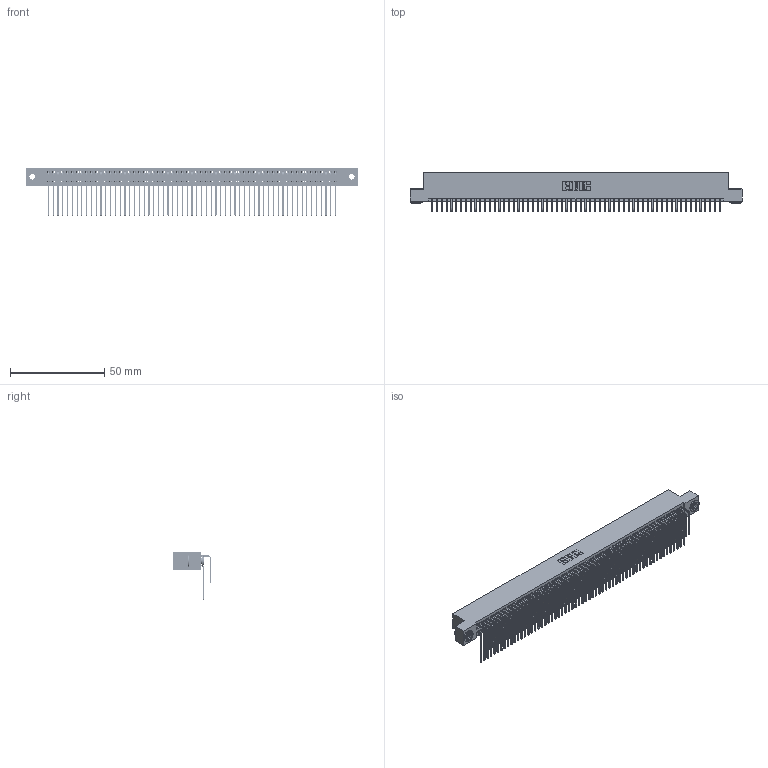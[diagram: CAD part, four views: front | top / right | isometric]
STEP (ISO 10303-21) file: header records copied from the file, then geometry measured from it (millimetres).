
FILE_DESCRIPTION (( 'STEP AP203' ), '1' );
FILE_NAME ('395-122-559-203.STEP', '2019-10-28T09:30:33', ( '' ), ( '' ), 'SwSTEP 2.0', 'SolidWorks 2016', '' );
FILE_SCHEMA (( 'CONFIG_CONTROL_DESIGN' ));
Length unit declared in the file: inch
Products named in the file (5): 345-250-002_345-250-002-102; 395-122-559-203; 345 Part_Flush Mounting Lugs - 0.156 Dia-TH; 345-292-001_558 559 Tail - 1; 345-292-001_559 Tail - 2
Assembly tree (125 placements, depth 2):
  395-122-559-203
    345 Part_Flush Mounting Lugs - 0.156 Dia-TH
    345-292-001_558 559 Tail - 1  x61
    345-292-001_559 Tail - 2  x61
    345-250-002_345-250-002-102  x2
Bounding box: 176.15 x 20.56 x 25.53 mm (x, y, z)
Volume: 18010.8 mm3; surface area: 30505.4 mm2
Topology: 125 solids, 125 shells, 6508 faces, 19327 edges, 12718 vertices
Faces by surface type: plane 4360, cylinder 2140, cone 8
Entity records: 47606 total; most frequent: CARTESIAN_POINT 7982, ORIENTED_EDGE 7858, DIRECTION 7019, EDGE_CURVE 3929, VECTOR 3489, LINE 3489, VERTEX_POINT 2614, AXIS2_PLACEMENT_3D 1765
